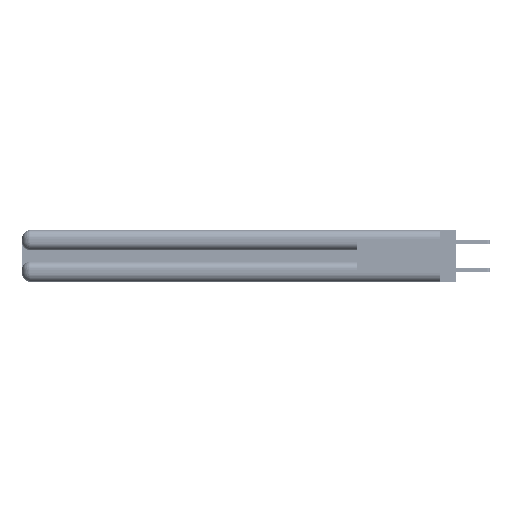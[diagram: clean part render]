
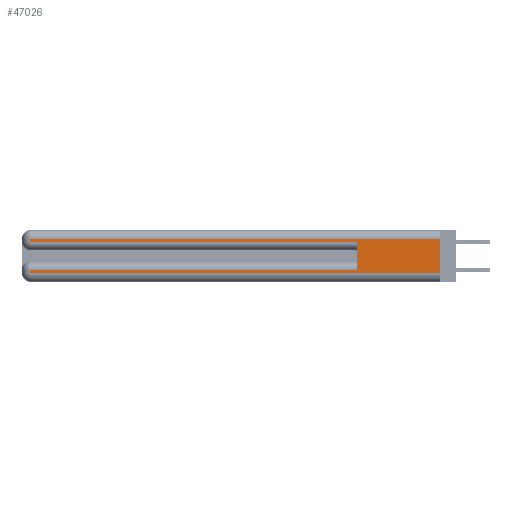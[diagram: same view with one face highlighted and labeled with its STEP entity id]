
A CAD part, left-side view. The second image highlights one B-rep face of the part: STEP entity #47026.
In plain terms, the highlighted planar face has unit normal (-1, 0, 0).
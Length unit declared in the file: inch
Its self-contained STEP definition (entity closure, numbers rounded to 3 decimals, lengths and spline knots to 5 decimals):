
#14 = CARTESIAN_POINT ( 'NONE',  ( 0., 2.94, 0.285 ) ) ;
#1345 = LINE ( 'NONE', #8554, #11311 ) ;
#1971 = DIRECTION ( 'NONE',  ( 0., 1., 0. ) ) ;
#2179 = ORIENTED_EDGE ( 'NONE', *, *, #49320, .F. ) ;
#2677 = EDGE_LOOP ( 'NONE', ( #19843, #23386, #29511, #48794, #2179, #24538, #17044, #49861 ) ) ;
#3911 = VERTEX_POINT ( 'NONE', #47433 ) ;
#3924 = CARTESIAN_POINT ( 'NONE',  ( 0., 2.94, 0.06 ) ) ;
#4259 = LINE ( 'NONE', #17155, #44950 ) ;
#6346 = CARTESIAN_POINT ( 'NONE',  ( 0., 2.94, 0.31 ) ) ;
#7829 = DIRECTION ( 'NONE',  ( 0., 1., 0. ) ) ;
#7971 = EDGE_CURVE ( 'NONE', #11639, #34453, #4259, .T. ) ;
#8554 = CARTESIAN_POINT ( 'NONE',  ( 0., 2.94, 0.37 ) ) ;
#9685 = FACE_OUTER_BOUND ( 'NONE', #2677, .T. ) ;
#11311 = VECTOR ( 'NONE', #21957, 39.37008 ) ;
#11639 = VERTEX_POINT ( 'NONE', #14 ) ;
#13060 = DIRECTION ( 'NONE',  ( 0., -1., 0. ) ) ;
#13320 = VERTEX_POINT ( 'NONE', #3924 ) ;
#13788 = AXIS2_PLACEMENT_3D ( 'NONE', #15597, #19864, #28833 ) ;
#14416 = CARTESIAN_POINT ( 'NONE',  ( 0., 0., 0.085 ) ) ;
#15597 = CARTESIAN_POINT ( 'NONE',  ( 0., 0., 0.37 ) ) ;
#16422 = VECTOR ( 'NONE', #38606, 39.37008 ) ;
#16764 = CARTESIAN_POINT ( 'NONE',  ( 0., 0., 0.06 ) ) ;
#17044 = ORIENTED_EDGE ( 'NONE', *, *, #38932, .T. ) ;
#17155 = CARTESIAN_POINT ( 'NONE',  ( 0., 0., 0.285 ) ) ;
#17923 = VERTEX_POINT ( 'NONE', #31133 ) ;
#19843 = ORIENTED_EDGE ( 'NONE', *, *, #50487, .F. ) ;
#19864 = DIRECTION ( 'NONE',  ( 1., 0., 0. ) ) ;
#21188 = CARTESIAN_POINT ( 'NONE',  ( 0., 2.94, 0.37 ) ) ;
#21461 = CARTESIAN_POINT ( 'NONE',  ( 0., 0.6, 0.145 ) ) ;
#21666 = LINE ( 'NONE', #47107, #32293 ) ;
#21957 = DIRECTION ( 'NONE',  ( 0., 0., -1. ) ) ;
#22118 = VERTEX_POINT ( 'NONE', #6346 ) ;
#22867 = LINE ( 'NONE', #14416, #32850 ) ;
#23386 = ORIENTED_EDGE ( 'NONE', *, *, #42959, .T. ) ;
#24538 = ORIENTED_EDGE ( 'NONE', *, *, #44147, .T. ) ;
#25169 = VERTEX_POINT ( 'NONE', #40720 ) ;
#25474 = DIRECTION ( 'NONE',  ( 0., 0., -1. ) ) ;
#25926 = CARTESIAN_POINT ( 'NONE',  ( 0., 0., 0.06 ) ) ;
#26111 = DIRECTION ( 'NONE',  ( 0., -1., 0. ) ) ;
#28833 = DIRECTION ( 'NONE',  ( 0., 0., -1. ) ) ;
#29511 = ORIENTED_EDGE ( 'NONE', *, *, #52984, .T. ) ;
#31133 = CARTESIAN_POINT ( 'NONE',  ( 0., 0.6, 0.085 ) ) ;
#32293 = VECTOR ( 'NONE', #47274, 39.37008 ) ;
#32850 = VECTOR ( 'NONE', #1971, 39.37008 ) ;
#33352 = CARTESIAN_POINT ( 'NONE',  ( 0., 0., 0.31 ) ) ;
#34453 = VERTEX_POINT ( 'NONE', #51623 ) ;
#38606 = DIRECTION ( 'NONE',  ( 0., 0., 1. ) ) ;
#38932 = EDGE_CURVE ( 'NONE', #3911, #13320, #1345, .T. ) ;
#40720 = CARTESIAN_POINT ( 'NONE',  ( 0., 0., 0.31 ) ) ;
#42959 = EDGE_CURVE ( 'NONE', #25169, #22118, #45725, .T. ) ;
#43189 = VERTEX_POINT ( 'NONE', #16764 ) ;
#43988 = VECTOR ( 'NONE', #26111, 39.37008 ) ;
#44147 = EDGE_CURVE ( 'NONE', #17923, #3911, #22867, .T. ) ;
#44468 = LINE ( 'NONE', #21461, #16422 ) ;
#44950 = VECTOR ( 'NONE', #13060, 39.37008 ) ;
#45725 = LINE ( 'NONE', #33352, #47682 ) ;
#45970 = EDGE_CURVE ( 'NONE', #13320, #43189, #49317, .T. ) ;
#46789 = VECTOR ( 'NONE', #25474, 39.37008 ) ;
#47026 = ADVANCED_FACE ( 'NONE', ( #9685 ), #54350, .F. ) ;
#47107 = CARTESIAN_POINT ( 'NONE',  ( 0., 0., 0.37 ) ) ;
#47274 = DIRECTION ( 'NONE',  ( 0., 0., -1. ) ) ;
#47433 = CARTESIAN_POINT ( 'NONE',  ( 0., 2.94, 0.085 ) ) ;
#47682 = VECTOR ( 'NONE', #7829, 39.37008 ) ;
#48794 = ORIENTED_EDGE ( 'NONE', *, *, #7971, .T. ) ;
#49317 = LINE ( 'NONE', #25926, #43988 ) ;
#49320 = EDGE_CURVE ( 'NONE', #17923, #34453, #44468, .T. ) ;
#49861 = ORIENTED_EDGE ( 'NONE', *, *, #45970, .T. ) ;
#50487 = EDGE_CURVE ( 'NONE', #25169, #43189, #21666, .T. ) ;
#51396 = LINE ( 'NONE', #21188, #46789 ) ;
#51623 = CARTESIAN_POINT ( 'NONE',  ( 0., 0.6, 0.285 ) ) ;
#52984 = EDGE_CURVE ( 'NONE', #22118, #11639, #51396, .T. ) ;
#54350 = PLANE ( 'NONE',  #13788 ) ;
